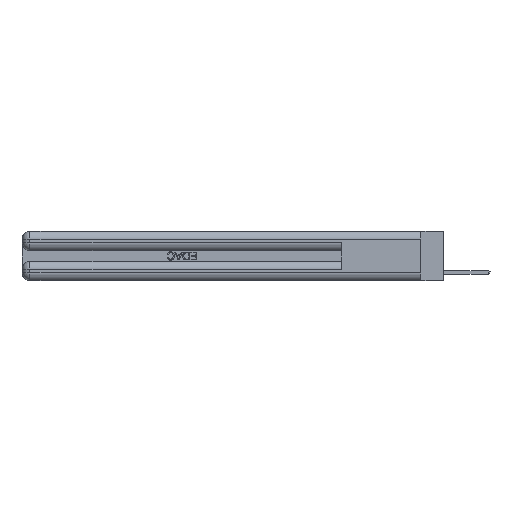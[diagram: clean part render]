
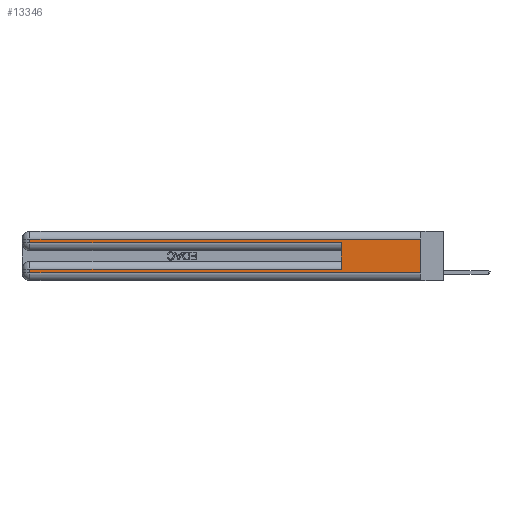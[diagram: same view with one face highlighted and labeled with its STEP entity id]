
A CAD part, left-side view. The second image highlights one B-rep face of the part: STEP entity #13346.
In plain terms, the highlighted planar face has unit normal (-1, 0, 0).
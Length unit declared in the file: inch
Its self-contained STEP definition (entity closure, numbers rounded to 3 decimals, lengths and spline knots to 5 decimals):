
#105 = ORIENTED_EDGE ( 'NONE', *, *, #3742, .T. ) ;
#335 = VERTEX_POINT ( 'NONE', #14306 ) ;
#869 = VERTEX_POINT ( 'NONE', #31649 ) ;
#1483 = VECTOR ( 'NONE', #29424, 39.37008 ) ;
#1712 = EDGE_CURVE ( 'NONE', #335, #22217, #24086, .T. ) ;
#1722 = VECTOR ( 'NONE', #3681, 39.37008 ) ;
#2050 = LINE ( 'NONE', #22274, #1483 ) ;
#2314 = DIRECTION ( 'NONE',  ( 0., 0., -1. ) ) ;
#2618 = DIRECTION ( 'NONE',  ( 1., 0., 0. ) ) ;
#2776 = CARTESIAN_POINT ( 'NONE',  ( 0., 0., 0.37 ) ) ;
#2793 = DIRECTION ( 'NONE',  ( 0., -1., 0. ) ) ;
#3096 = DIRECTION ( 'NONE',  ( 0., 0., -1. ) ) ;
#3511 = CARTESIAN_POINT ( 'NONE',  ( 0., 2.94, 0.37 ) ) ;
#3622 = EDGE_CURVE ( 'NONE', #18773, #30797, #20060, .T. ) ;
#3681 = DIRECTION ( 'NONE',  ( 0., 0., -1. ) ) ;
#3742 = EDGE_CURVE ( 'NONE', #22217, #869, #23197, .T. ) ;
#4627 = VECTOR ( 'NONE', #10464, 39.37008 ) ;
#5425 = PLANE ( 'NONE',  #12320 ) ;
#6576 = CARTESIAN_POINT ( 'NONE',  ( 0., 0., 0.06 ) ) ;
#6727 = ORIENTED_EDGE ( 'NONE', *, *, #21701, .T. ) ;
#8250 = CARTESIAN_POINT ( 'NONE',  ( 0., 0., 0.285 ) ) ;
#10451 = ORIENTED_EDGE ( 'NONE', *, *, #24389, .T. ) ;
#10464 = DIRECTION ( 'NONE',  ( 0., -1., 0. ) ) ;
#11511 = CARTESIAN_POINT ( 'NONE',  ( 0., 0.6, 0.145 ) ) ;
#11557 = VERTEX_POINT ( 'NONE', #6576 ) ;
#11834 = VERTEX_POINT ( 'NONE', #12853 ) ;
#12064 = VECTOR ( 'NONE', #2793, 39.37008 ) ;
#12320 = AXIS2_PLACEMENT_3D ( 'NONE', #2776, #2618, #3096 ) ;
#12853 = CARTESIAN_POINT ( 'NONE',  ( 0., 0.6, 0.085 ) ) ;
#13346 = ADVANCED_FACE ( 'NONE', ( #28159 ), #5425, .F. ) ;
#13899 = LINE ( 'NONE', #21365, #4627 ) ;
#14306 = CARTESIAN_POINT ( 'NONE',  ( 0., 2.94, 0.31 ) ) ;
#14449 = DIRECTION ( 'NONE',  ( 0., 1., 0. ) ) ;
#15899 = LINE ( 'NONE', #11511, #18421 ) ;
#17113 = LINE ( 'NONE', #24562, #30475 ) ;
#17696 = CARTESIAN_POINT ( 'NONE',  ( 0., 2.94, 0.085 ) ) ;
#18421 = VECTOR ( 'NONE', #20868, 39.37008 ) ;
#18773 = VERTEX_POINT ( 'NONE', #17696 ) ;
#20060 = LINE ( 'NONE', #30198, #31678 ) ;
#20477 = VECTOR ( 'NONE', #14449, 39.37008 ) ;
#20868 = DIRECTION ( 'NONE',  ( 0., 0., 1. ) ) ;
#21237 = EDGE_LOOP ( 'NONE', ( #24128, #6727, #31063, #105, #30187, #25505, #25963, #10451 ) ) ;
#21365 = CARTESIAN_POINT ( 'NONE',  ( 0., 0., 0.06 ) ) ;
#21701 = EDGE_CURVE ( 'NONE', #28869, #335, #17113, .T. ) ;
#22087 = CARTESIAN_POINT ( 'NONE',  ( 0., 0., 0.085 ) ) ;
#22217 = VERTEX_POINT ( 'NONE', #32168 ) ;
#22274 = CARTESIAN_POINT ( 'NONE',  ( 0., 0., 0.37 ) ) ;
#23197 = LINE ( 'NONE', #8250, #12064 ) ;
#24086 = LINE ( 'NONE', #3511, #1722 ) ;
#24128 = ORIENTED_EDGE ( 'NONE', *, *, #24725, .F. ) ;
#24389 = EDGE_CURVE ( 'NONE', #30797, #11557, #13899, .T. ) ;
#24562 = CARTESIAN_POINT ( 'NONE',  ( 0., 0., 0.31 ) ) ;
#24725 = EDGE_CURVE ( 'NONE', #28869, #11557, #2050, .T. ) ;
#25342 = CARTESIAN_POINT ( 'NONE',  ( 0., 0., 0.31 ) ) ;
#25505 = ORIENTED_EDGE ( 'NONE', *, *, #29726, .T. ) ;
#25963 = ORIENTED_EDGE ( 'NONE', *, *, #3622, .T. ) ;
#26723 = DIRECTION ( 'NONE',  ( 0., 1., 0. ) ) ;
#27079 = LINE ( 'NONE', #22087, #20477 ) ;
#28159 = FACE_OUTER_BOUND ( 'NONE', #21237, .T. ) ;
#28869 = VERTEX_POINT ( 'NONE', #25342 ) ;
#29424 = DIRECTION ( 'NONE',  ( 0., 0., -1. ) ) ;
#29726 = EDGE_CURVE ( 'NONE', #11834, #18773, #27079, .T. ) ;
#30187 = ORIENTED_EDGE ( 'NONE', *, *, #31598, .F. ) ;
#30198 = CARTESIAN_POINT ( 'NONE',  ( 0., 2.94, 0.37 ) ) ;
#30428 = CARTESIAN_POINT ( 'NONE',  ( 0., 2.94, 0.06 ) ) ;
#30475 = VECTOR ( 'NONE', #26723, 39.37008 ) ;
#30797 = VERTEX_POINT ( 'NONE', #30428 ) ;
#31063 = ORIENTED_EDGE ( 'NONE', *, *, #1712, .T. ) ;
#31598 = EDGE_CURVE ( 'NONE', #11834, #869, #15899, .T. ) ;
#31649 = CARTESIAN_POINT ( 'NONE',  ( 0., 0.6, 0.285 ) ) ;
#31678 = VECTOR ( 'NONE', #2314, 39.37008 ) ;
#32168 = CARTESIAN_POINT ( 'NONE',  ( 0., 2.94, 0.285 ) ) ;
